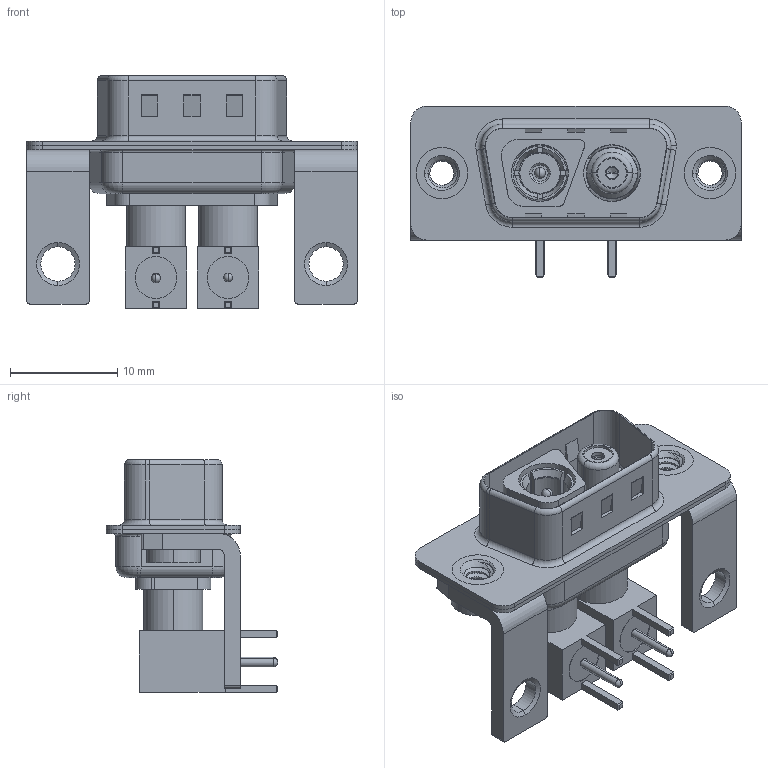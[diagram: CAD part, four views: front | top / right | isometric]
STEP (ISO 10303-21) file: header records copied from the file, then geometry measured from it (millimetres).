
FILE_DESCRIPTION (( 'STEP AP203' ), '1' );
FILE_NAME ('629-2WK2240-5NC.STEP', '2022-05-04T23:21:54', ( '' ), ( '' ), 'SwSTEP 2.0', 'SolidWorks 2020', '' );
FILE_SCHEMA (( 'CONFIG_CONTROL_DESIGN' ));
Length unit declared in the file: millimetre
Products named in the file (18): 629Combo Threaded Rivet_2; Insulator Socket; 629Combo Shell Rear_09 Contacts; RA Back Shell; Pin_RA; 629Combo Shell Front_09 Contacts; Co-Ax Plug Assy_RA; 629Combo Housing_2WK2; Insulator Socket 2; Insulator Pin_Straight PC Tail; 629-2WK2240-5NC; 629Combo Stabilizer Bracket; Co-Ax Plug_RA PC Tail; Co-Ax Jack Assy_RA; Co-Ax Jack_RA PC Tail; Locking Collar; Socket_RA; Insulator RA Pin
Assembly tree (22 placements, depth 3):
  629-2WK2240-5NC
    629Combo Housing_2WK2
    629Combo Shell Rear_09 Contacts
    629Combo Shell Front_09 Contacts
    629Combo Threaded Rivet_2  x2
    629Combo Stabilizer Bracket  x2
    Co-Ax Plug Assy_RA
      Co-Ax Plug_RA PC Tail
      Insulator Pin_Straight PC Tail
      Pin_RA
      Locking Collar
      RA Back Shell
      Insulator RA Pin
    Co-Ax Jack Assy_RA
      Co-Ax Jack_RA PC Tail
      Insulator Socket
      Insulator Socket 2
      Locking Collar
      Socket_RA
      RA Back Shell
      Insulator RA Pin
Bounding box: 30.8 x 16 x 21.71 mm (x, y, z)
Volume: 2305.1 mm3; surface area: 6241.8 mm2
Topology: 20 solids, 20 shells, 682 faces, 1658 edges, 1040 vertices
Faces by surface type: cylinder 290, plane 256, torus 62, cone 60, bspline 8, sphere 6
Entity records: 20362 total; most frequent: CARTESIAN_POINT 4634, DIRECTION 3071, ORIENTED_EDGE 2720, EDGE_CURVE 1360, AXIS2_PLACEMENT_3D 1201, VERTEX_POINT 861, LINE 669, VECTOR 669
